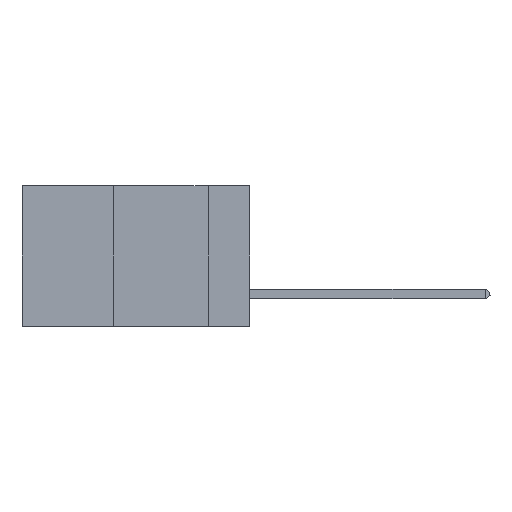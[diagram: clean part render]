
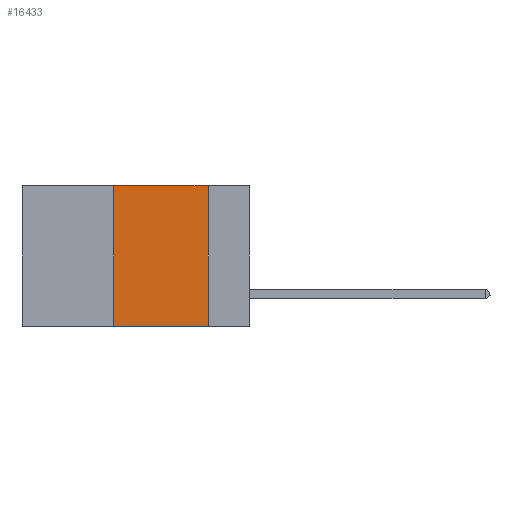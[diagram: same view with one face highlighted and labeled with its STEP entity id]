
A CAD part, left-side view. The second image highlights one B-rep face of the part: STEP entity #16433.
In plain terms, the highlighted planar face has unit normal (-1, 0, 0).
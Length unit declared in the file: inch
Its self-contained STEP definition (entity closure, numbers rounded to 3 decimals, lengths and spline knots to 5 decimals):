
#284 = VERTEX_POINT ( 'NONE', #725 ) ;
#725 = CARTESIAN_POINT ( 'NONE',  ( 0., 0.11, -0.37 ) ) ;
#970 = LINE ( 'NONE', #1668, #13143 ) ;
#1668 = CARTESIAN_POINT ( 'NONE',  ( 0., 0.6, 0. ) ) ;
#1782 = CARTESIAN_POINT ( 'NONE',  ( 0., 0.6, -0.37 ) ) ;
#2290 = ORIENTED_EDGE ( 'NONE', *, *, #33357, .F. ) ;
#2692 = AXIS2_PLACEMENT_3D ( 'NONE', #33186, #21966, #20072 ) ;
#6295 = CARTESIAN_POINT ( 'NONE',  ( 0., 0.36, 0. ) ) ;
#6402 = EDGE_CURVE ( 'NONE', #13601, #28431, #970, .T. ) ;
#6806 = DIRECTION ( 'NONE',  ( 0., -1., 0. ) ) ;
#8843 = VECTOR ( 'NONE', #17811, 39.37008 ) ;
#9185 = ORIENTED_EDGE ( 'NONE', *, *, #17956, .T. ) ;
#9558 = FACE_OUTER_BOUND ( 'NONE', #19756, .T. ) ;
#10978 = CARTESIAN_POINT ( 'NONE',  ( 0., 0.11, 0. ) ) ;
#12440 = LINE ( 'NONE', #30396, #8843 ) ;
#12628 = LINE ( 'NONE', #20394, #13936 ) ;
#13143 = VECTOR ( 'NONE', #6806, 39.37008 ) ;
#13601 = VERTEX_POINT ( 'NONE', #6295 ) ;
#13936 = VECTOR ( 'NONE', #30928, 39.37008 ) ;
#16433 = ADVANCED_FACE ( 'NONE', ( #9558 ), #27677, .F. ) ;
#17811 = DIRECTION ( 'NONE',  ( 0., 0., 1. ) ) ;
#17956 = EDGE_CURVE ( 'NONE', #27119, #284, #25368, .T. ) ;
#18741 = CARTESIAN_POINT ( 'NONE',  ( 0., 0.36, -0.37 ) ) ;
#19756 = EDGE_LOOP ( 'NONE', ( #2290, #22159, #28990, #9185 ) ) ;
#20072 = DIRECTION ( 'NONE',  ( 0., 0., -1. ) ) ;
#20394 = CARTESIAN_POINT ( 'NONE',  ( 0., 0.11, 0. ) ) ;
#21966 = DIRECTION ( 'NONE',  ( 1., 0., 0. ) ) ;
#22159 = ORIENTED_EDGE ( 'NONE', *, *, #6402, .F. ) ;
#25368 = LINE ( 'NONE', #1782, #26426 ) ;
#26426 = VECTOR ( 'NONE', #32946, 39.37008 ) ;
#27119 = VERTEX_POINT ( 'NONE', #18741 ) ;
#27677 = PLANE ( 'NONE',  #2692 ) ;
#28431 = VERTEX_POINT ( 'NONE', #10978 ) ;
#28990 = ORIENTED_EDGE ( 'NONE', *, *, #30449, .F. ) ;
#30396 = CARTESIAN_POINT ( 'NONE',  ( 0., 0.36, 0. ) ) ;
#30449 = EDGE_CURVE ( 'NONE', #27119, #13601, #12440, .T. ) ;
#30928 = DIRECTION ( 'NONE',  ( 0., 0., -1. ) ) ;
#32946 = DIRECTION ( 'NONE',  ( 0., -1., 0. ) ) ;
#33186 = CARTESIAN_POINT ( 'NONE',  ( 0., 0.6, 0. ) ) ;
#33357 = EDGE_CURVE ( 'NONE', #28431, #284, #12628, .T. ) ;
